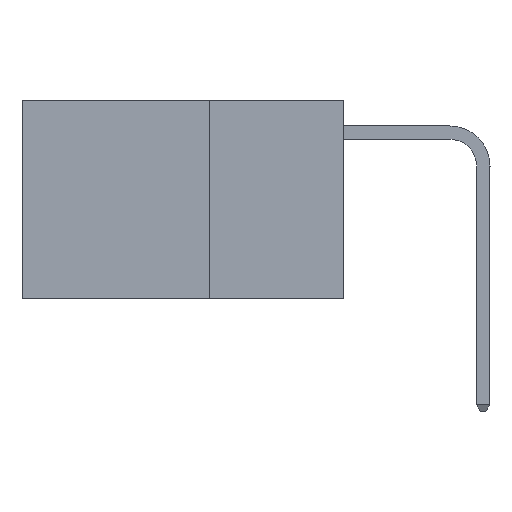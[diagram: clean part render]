
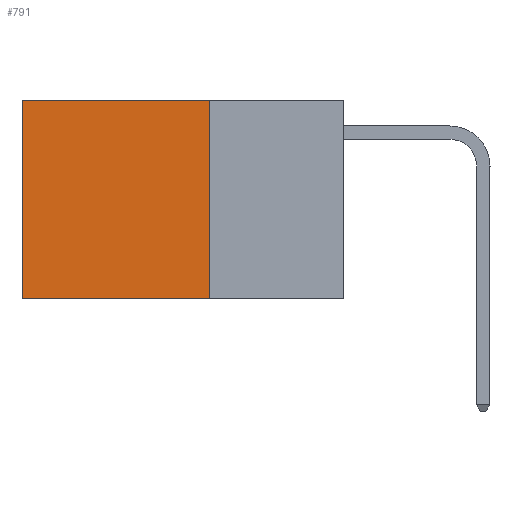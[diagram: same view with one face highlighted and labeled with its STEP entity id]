
A CAD part, left-side view. The second image highlights one B-rep face of the part: STEP entity #791.
In plain terms, the highlighted planar face has unit normal (-1, 0, 0).
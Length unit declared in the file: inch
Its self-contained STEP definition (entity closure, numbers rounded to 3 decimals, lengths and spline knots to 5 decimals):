
#141 = CARTESIAN_POINT ( 'NONE',  ( 0.2625, 0.25, 0. ) ) ;
#650 = LINE ( 'NONE', #24580, #16851 ) ;
#791 = ADVANCED_FACE ( 'NONE', ( #23677 ), #20550, .F. ) ;
#1119 = CARTESIAN_POINT ( 'NONE',  ( 0.2625, 0.25, -0.37 ) ) ;
#2850 = VERTEX_POINT ( 'NONE', #3718 ) ;
#3286 = DIRECTION ( 'NONE',  ( 0., 1., 0. ) ) ;
#3718 = CARTESIAN_POINT ( 'NONE',  ( 0.2625, 0.25, -0.37 ) ) ;
#3729 = CARTESIAN_POINT ( 'NONE',  ( 0.2625, 0.6, 0. ) ) ;
#3792 = ORIENTED_EDGE ( 'NONE', *, *, #13042, .T. ) ;
#5317 = VERTEX_POINT ( 'NONE', #141 ) ;
#5377 = VERTEX_POINT ( 'NONE', #3729 ) ;
#7609 = VERTEX_POINT ( 'NONE', #13758 ) ;
#8183 = ORIENTED_EDGE ( 'NONE', *, *, #27012, .T. ) ;
#8669 = LINE ( 'NONE', #15600, #14254 ) ;
#9273 = DIRECTION ( 'NONE',  ( 0., 0., -1. ) ) ;
#9675 = EDGE_CURVE ( 'NONE', #2850, #7609, #18506, .T. ) ;
#10045 = DIRECTION ( 'NONE',  ( 0., 0., -1. ) ) ;
#11585 = CARTESIAN_POINT ( 'NONE',  ( 0.2625, 0.25, 0. ) ) ;
#11983 = EDGE_LOOP ( 'NONE', ( #8183, #17423, #16071, #3792 ) ) ;
#12323 = VECTOR ( 'NONE', #3286, 39.37008 ) ;
#12677 = VECTOR ( 'NONE', #26060, 39.37008 ) ;
#13042 = EDGE_CURVE ( 'NONE', #5317, #5377, #23683, .T. ) ;
#13758 = CARTESIAN_POINT ( 'NONE',  ( 0.2625, 0.6, -0.37 ) ) ;
#14254 = VECTOR ( 'NONE', #9273, 39.37008 ) ;
#15013 = EDGE_CURVE ( 'NONE', #5317, #2850, #650, .T. ) ;
#15600 = CARTESIAN_POINT ( 'NONE',  ( 0.2625, 0.6, 0. ) ) ;
#16071 = ORIENTED_EDGE ( 'NONE', *, *, #15013, .F. ) ;
#16851 = VECTOR ( 'NONE', #10045, 39.37008 ) ;
#17423 = ORIENTED_EDGE ( 'NONE', *, *, #9675, .F. ) ;
#18506 = LINE ( 'NONE', #1119, #12323 ) ;
#20273 = DIRECTION ( 'NONE',  ( 0., 0., -1. ) ) ;
#20296 = DIRECTION ( 'NONE',  ( 1., 0., 0. ) ) ;
#20364 = CARTESIAN_POINT ( 'NONE',  ( 0.2625, 0.25, 0. ) ) ;
#20550 = PLANE ( 'NONE',  #23807 ) ;
#23677 = FACE_OUTER_BOUND ( 'NONE', #11983, .T. ) ;
#23683 = LINE ( 'NONE', #11585, #12677 ) ;
#23807 = AXIS2_PLACEMENT_3D ( 'NONE', #20364, #20296, #20273 ) ;
#24580 = CARTESIAN_POINT ( 'NONE',  ( 0.2625, 0.25, 0. ) ) ;
#26060 = DIRECTION ( 'NONE',  ( 0., 1., 0. ) ) ;
#27012 = EDGE_CURVE ( 'NONE', #5377, #7609, #8669, .T. ) ;
